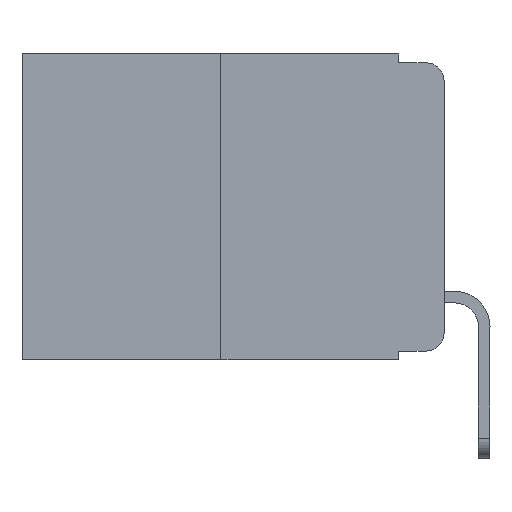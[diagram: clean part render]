
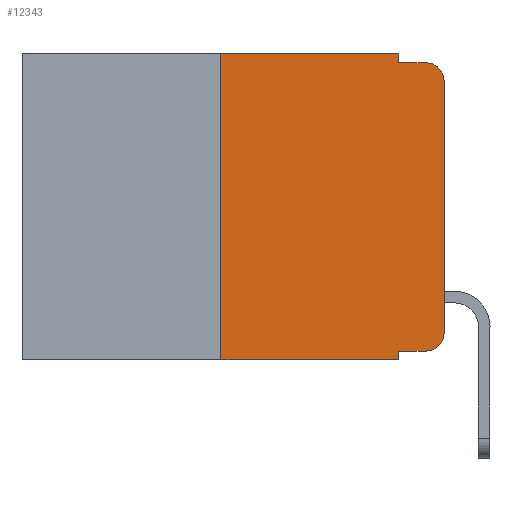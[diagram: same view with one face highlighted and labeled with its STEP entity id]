
A CAD part, left-side view. The second image highlights one B-rep face of the part: STEP entity #12343.
In plain terms, the highlighted planar face has unit normal (-1, 0, 0).
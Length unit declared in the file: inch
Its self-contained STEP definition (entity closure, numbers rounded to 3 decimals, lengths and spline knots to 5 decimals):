
#81 = LINE ( 'NONE', #402, #14221 ) ;
#322 = CARTESIAN_POINT ( 'NONE',  ( 0., 0.02, -0.01 ) ) ;
#402 = CARTESIAN_POINT ( 'NONE',  ( 0., 0., 0. ) ) ;
#481 = DIRECTION ( 'NONE',  ( 0., 0., -1. ) ) ;
#602 = CIRCLE ( 'NONE', #1497, 0.02 ) ;
#804 = LINE ( 'NONE', #9631, #10716 ) ;
#919 = VERTEX_POINT ( 'NONE', #11692 ) ;
#1088 = EDGE_CURVE ( 'NONE', #4690, #15425, #804, .T. ) ;
#1089 = CARTESIAN_POINT ( 'NONE',  ( 0., 0.473, 0. ) ) ;
#1148 = DIRECTION ( 'NONE',  ( 0., -1., 0. ) ) ;
#1208 = CARTESIAN_POINT ( 'NONE',  ( 0., 0.25, 0. ) ) ;
#1388 = CARTESIAN_POINT ( 'NONE',  ( 0., 0.473, -0.343 ) ) ;
#1497 = AXIS2_PLACEMENT_3D ( 'NONE', #10780, #1979, #481 ) ;
#1613 = EDGE_CURVE ( 'NONE', #15808, #15425, #602, .T. ) ;
#1921 = LINE ( 'NONE', #1388, #3925 ) ;
#1979 = DIRECTION ( 'NONE',  ( -1., 0., 0. ) ) ;
#2172 = EDGE_LOOP ( 'NONE', ( #8185, #9921, #9037, #3723, #8368, #11379, #16504, #9310, #7743, #6949 ) ) ;
#2232 = EDGE_CURVE ( 'NONE', #16000, #13999, #11208, .T. ) ;
#2321 = VECTOR ( 'NONE', #8965, 39.37008 ) ;
#2390 = CARTESIAN_POINT ( 'NONE',  ( 0., 0.051, -0.343 ) ) ;
#3641 = CARTESIAN_POINT ( 'NONE',  ( 0., 0.051, -0.333 ) ) ;
#3723 = ORIENTED_EDGE ( 'NONE', *, *, #9116, .F. ) ;
#3925 = VECTOR ( 'NONE', #5102, 39.37008 ) ;
#4258 = CARTESIAN_POINT ( 'NONE',  ( 0., 0.473, 0. ) ) ;
#4690 = VERTEX_POINT ( 'NONE', #16217 ) ;
#4701 = DIRECTION ( 'NONE',  ( 0., 0., 1. ) ) ;
#4899 = CARTESIAN_POINT ( 'NONE',  ( 0., 0.25, -0.343 ) ) ;
#5102 = DIRECTION ( 'NONE',  ( 0., -1., 0. ) ) ;
#6929 = VECTOR ( 'NONE', #16584, 39.37008 ) ;
#6949 = ORIENTED_EDGE ( 'NONE', *, *, #7482, .T. ) ;
#7064 = AXIS2_PLACEMENT_3D ( 'NONE', #4258, #14394, #13284 ) ;
#7266 = CARTESIAN_POINT ( 'NONE',  ( 0., 0.02, -0.333 ) ) ;
#7387 = LINE ( 'NONE', #16692, #2321 ) ;
#7409 = VECTOR ( 'NONE', #1148, 39.37008 ) ;
#7482 = EDGE_CURVE ( 'NONE', #15077, #919, #12640, .T. ) ;
#7664 = VERTEX_POINT ( 'NONE', #14842 ) ;
#7687 = CARTESIAN_POINT ( 'NONE',  ( 0., 0., -0.03 ) ) ;
#7743 = ORIENTED_EDGE ( 'NONE', *, *, #7988, .T. ) ;
#7785 = VECTOR ( 'NONE', #4701, 39.37008 ) ;
#7968 = DIRECTION ( 'NONE',  ( 0., 0., -1. ) ) ;
#7988 = EDGE_CURVE ( 'NONE', #11066, #15077, #7387, .T. ) ;
#8097 = DIRECTION ( 'NONE',  ( 0., 0., -1. ) ) ;
#8185 = ORIENTED_EDGE ( 'NONE', *, *, #12374, .T. ) ;
#8368 = ORIENTED_EDGE ( 'NONE', *, *, #15146, .F. ) ;
#8526 = AXIS2_PLACEMENT_3D ( 'NONE', #14408, #9443, #7968 ) ;
#8965 = DIRECTION ( 'NONE',  ( 0., -1., 0. ) ) ;
#9037 = ORIENTED_EDGE ( 'NONE', *, *, #1088, .F. ) ;
#9116 = EDGE_CURVE ( 'NONE', #7664, #4690, #11760, .T. ) ;
#9310 = ORIENTED_EDGE ( 'NONE', *, *, #10600, .F. ) ;
#9312 = VERTEX_POINT ( 'NONE', #2390 ) ;
#9443 = DIRECTION ( 'NONE',  ( -1., 0., 0. ) ) ;
#9483 = DIRECTION ( 'NONE',  ( 0., 0., 1. ) ) ;
#9631 = CARTESIAN_POINT ( 'NONE',  ( 0., 0.051, -0.01 ) ) ;
#9632 = FACE_OUTER_BOUND ( 'NONE', #2172, .T. ) ;
#9825 = VECTOR ( 'NONE', #8097, 39.37008 ) ;
#9921 = ORIENTED_EDGE ( 'NONE', *, *, #1613, .T. ) ;
#10600 = EDGE_CURVE ( 'NONE', #11066, #9312, #11627, .T. ) ;
#10716 = VECTOR ( 'NONE', #15764, 39.37008 ) ;
#10780 = CARTESIAN_POINT ( 'NONE',  ( 0., 0.02, -0.03 ) ) ;
#11066 = VERTEX_POINT ( 'NONE', #3641 ) ;
#11208 = LINE ( 'NONE', #16410, #7785 ) ;
#11379 = ORIENTED_EDGE ( 'NONE', *, *, #2232, .F. ) ;
#11627 = LINE ( 'NONE', #15670, #9825 ) ;
#11692 = CARTESIAN_POINT ( 'NONE',  ( 0., 0., -0.313 ) ) ;
#11760 = LINE ( 'NONE', #13944, #6929 ) ;
#12343 = ADVANCED_FACE ( 'NONE', ( #9632 ), #13340, .F. ) ;
#12374 = EDGE_CURVE ( 'NONE', #919, #15808, #81, .T. ) ;
#12640 = CIRCLE ( 'NONE', #8526, 0.02 ) ;
#13284 = DIRECTION ( 'NONE',  ( 0., 0., -1. ) ) ;
#13340 = PLANE ( 'NONE',  #7064 ) ;
#13944 = CARTESIAN_POINT ( 'NONE',  ( 0., 0.051, 0. ) ) ;
#13999 = VERTEX_POINT ( 'NONE', #1208 ) ;
#14221 = VECTOR ( 'NONE', #9483, 39.37008 ) ;
#14394 = DIRECTION ( 'NONE',  ( 1., 0., 0. ) ) ;
#14408 = CARTESIAN_POINT ( 'NONE',  ( 0., 0.02, -0.313 ) ) ;
#14842 = CARTESIAN_POINT ( 'NONE',  ( 0., 0.051, 0. ) ) ;
#15077 = VERTEX_POINT ( 'NONE', #7266 ) ;
#15146 = EDGE_CURVE ( 'NONE', #13999, #7664, #15845, .T. ) ;
#15425 = VERTEX_POINT ( 'NONE', #322 ) ;
#15670 = CARTESIAN_POINT ( 'NONE',  ( 0., 0.051, 0. ) ) ;
#15764 = DIRECTION ( 'NONE',  ( 0., -1., 0. ) ) ;
#15808 = VERTEX_POINT ( 'NONE', #7687 ) ;
#15845 = LINE ( 'NONE', #1089, #7409 ) ;
#16000 = VERTEX_POINT ( 'NONE', #4899 ) ;
#16076 = EDGE_CURVE ( 'NONE', #16000, #9312, #1921, .T. ) ;
#16217 = CARTESIAN_POINT ( 'NONE',  ( 0., 0.051, -0.01 ) ) ;
#16410 = CARTESIAN_POINT ( 'NONE',  ( 0., 0.25, 0. ) ) ;
#16504 = ORIENTED_EDGE ( 'NONE', *, *, #16076, .T. ) ;
#16584 = DIRECTION ( 'NONE',  ( 0., 0., -1. ) ) ;
#16692 = CARTESIAN_POINT ( 'NONE',  ( 0., 0.051, -0.333 ) ) ;
